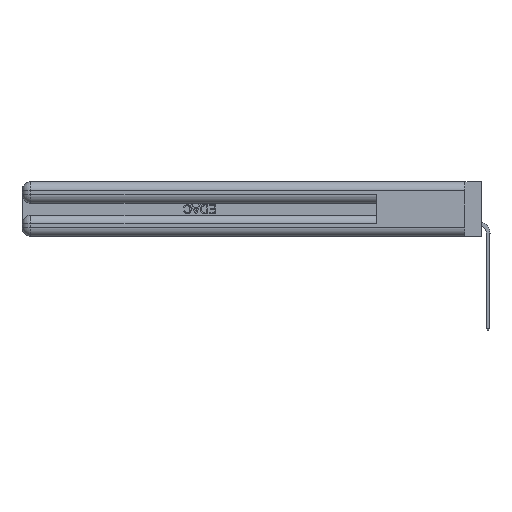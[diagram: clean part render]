
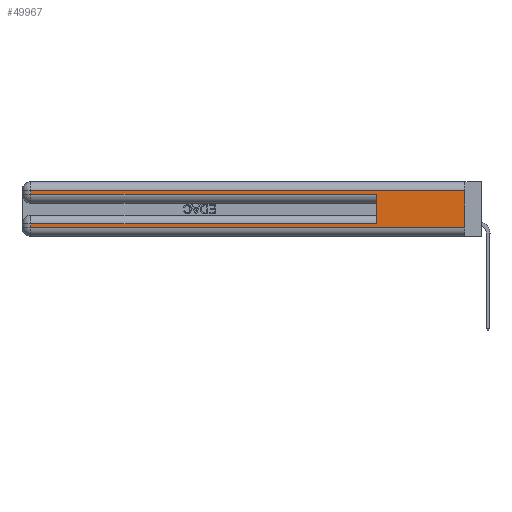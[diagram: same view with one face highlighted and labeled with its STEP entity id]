
A CAD part, left-side view. The second image highlights one B-rep face of the part: STEP entity #49967.
In plain terms, the highlighted planar face has unit normal (-1, 0, 0).
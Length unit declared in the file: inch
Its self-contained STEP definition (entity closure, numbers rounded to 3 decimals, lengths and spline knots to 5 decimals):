
#33 = CARTESIAN_POINT ( 'NONE',  ( 0., 2.94, 0.06 ) ) ;
#1053 = VERTEX_POINT ( 'NONE', #41609 ) ;
#1568 = VECTOR ( 'NONE', #34694, 39.37008 ) ;
#3211 = CARTESIAN_POINT ( 'NONE',  ( 0., 2.94, 0.37 ) ) ;
#3875 = DIRECTION ( 'NONE',  ( 0., 0., -1. ) ) ;
#4368 = EDGE_CURVE ( 'NONE', #27882, #26695, #31120, .T. ) ;
#5162 = LINE ( 'NONE', #8670, #21105 ) ;
#5306 = EDGE_CURVE ( 'NONE', #41147, #31050, #9537, .T. ) ;
#5658 = VERTEX_POINT ( 'NONE', #22631 ) ;
#6434 = ORIENTED_EDGE ( 'NONE', *, *, #20993, .F. ) ;
#6780 = ORIENTED_EDGE ( 'NONE', *, *, #15509, .T. ) ;
#6915 = DIRECTION ( 'NONE',  ( 1., 0., 0. ) ) ;
#7649 = DIRECTION ( 'NONE',  ( 0., 0., -1. ) ) ;
#8670 = CARTESIAN_POINT ( 'NONE',  ( 0., 0.6, 0.145 ) ) ;
#9537 = LINE ( 'NONE', #39548, #12088 ) ;
#10649 = EDGE_CURVE ( 'NONE', #43147, #5658, #30292, .T. ) ;
#11009 = CARTESIAN_POINT ( 'NONE',  ( 0., 0., 0.37 ) ) ;
#11147 = ORIENTED_EDGE ( 'NONE', *, *, #10649, .T. ) ;
#12088 = VECTOR ( 'NONE', #47652, 39.37008 ) ;
#12813 = EDGE_CURVE ( 'NONE', #22686, #1053, #13637, .T. ) ;
#13637 = LINE ( 'NONE', #44095, #20621 ) ;
#14068 = ORIENTED_EDGE ( 'NONE', *, *, #35236, .F. ) ;
#15509 = EDGE_CURVE ( 'NONE', #31050, #27882, #30389, .T. ) ;
#17684 = CARTESIAN_POINT ( 'NONE',  ( 0., 2.94, 0.31 ) ) ;
#18006 = ORIENTED_EDGE ( 'NONE', *, *, #21925, .T. ) ;
#18029 = LINE ( 'NONE', #46171, #1568 ) ;
#18908 = ORIENTED_EDGE ( 'NONE', *, *, #12813, .T. ) ;
#19089 = VECTOR ( 'NONE', #47805, 39.37008 ) ;
#19190 = CARTESIAN_POINT ( 'NONE',  ( 0., 2.94, 0.285 ) ) ;
#19454 = CARTESIAN_POINT ( 'NONE',  ( 0., 0., 0.285 ) ) ;
#19602 = DIRECTION ( 'NONE',  ( 0., 1., 0. ) ) ;
#20621 = VECTOR ( 'NONE', #19602, 39.37008 ) ;
#20917 = DIRECTION ( 'NONE',  ( 0., -1., 0. ) ) ;
#20993 = EDGE_CURVE ( 'NONE', #41147, #5658, #18029, .T. ) ;
#21105 = VECTOR ( 'NONE', #49849, 39.37008 ) ;
#21925 = EDGE_CURVE ( 'NONE', #1053, #43147, #50861, .T. ) ;
#22631 = CARTESIAN_POINT ( 'NONE',  ( 0., 0., 0.06 ) ) ;
#22686 = VERTEX_POINT ( 'NONE', #48046 ) ;
#23017 = DIRECTION ( 'NONE',  ( 0., 0., -1. ) ) ;
#26695 = VERTEX_POINT ( 'NONE', #37010 ) ;
#27882 = VERTEX_POINT ( 'NONE', #19190 ) ;
#30292 = LINE ( 'NONE', #47527, #32253 ) ;
#30389 = LINE ( 'NONE', #38270, #50641 ) ;
#31050 = VERTEX_POINT ( 'NONE', #17684 ) ;
#31120 = LINE ( 'NONE', #19454, #19089 ) ;
#32253 = VECTOR ( 'NONE', #20917, 39.37008 ) ;
#32547 = VECTOR ( 'NONE', #3875, 39.37008 ) ;
#34694 = DIRECTION ( 'NONE',  ( 0., 0., -1. ) ) ;
#35236 = EDGE_CURVE ( 'NONE', #22686, #26695, #5162, .T. ) ;
#35499 = ORIENTED_EDGE ( 'NONE', *, *, #4368, .T. ) ;
#37010 = CARTESIAN_POINT ( 'NONE',  ( 0., 0.6, 0.285 ) ) ;
#37459 = ORIENTED_EDGE ( 'NONE', *, *, #5306, .T. ) ;
#38270 = CARTESIAN_POINT ( 'NONE',  ( 0., 2.94, 0.37 ) ) ;
#39548 = CARTESIAN_POINT ( 'NONE',  ( 0., 0., 0.31 ) ) ;
#39807 = FACE_OUTER_BOUND ( 'NONE', #52107, .T. ) ;
#41147 = VERTEX_POINT ( 'NONE', #50049 ) ;
#41609 = CARTESIAN_POINT ( 'NONE',  ( 0., 2.94, 0.085 ) ) ;
#43147 = VERTEX_POINT ( 'NONE', #33 ) ;
#44095 = CARTESIAN_POINT ( 'NONE',  ( 0., 0., 0.085 ) ) ;
#46171 = CARTESIAN_POINT ( 'NONE',  ( 0., 0., 0.37 ) ) ;
#47527 = CARTESIAN_POINT ( 'NONE',  ( 0., 0., 0.06 ) ) ;
#47652 = DIRECTION ( 'NONE',  ( 0., 1., 0. ) ) ;
#47805 = DIRECTION ( 'NONE',  ( 0., -1., 0. ) ) ;
#48046 = CARTESIAN_POINT ( 'NONE',  ( 0., 0.6, 0.085 ) ) ;
#49849 = DIRECTION ( 'NONE',  ( 0., 0., 1. ) ) ;
#49967 = ADVANCED_FACE ( 'NONE', ( #39807 ), #51337, .F. ) ;
#50049 = CARTESIAN_POINT ( 'NONE',  ( 0., 0., 0.31 ) ) ;
#50641 = VECTOR ( 'NONE', #23017, 39.37008 ) ;
#50861 = LINE ( 'NONE', #3211, #32547 ) ;
#51337 = PLANE ( 'NONE',  #52116 ) ;
#52107 = EDGE_LOOP ( 'NONE', ( #6434, #37459, #6780, #35499, #14068, #18908, #18006, #11147 ) ) ;
#52116 = AXIS2_PLACEMENT_3D ( 'NONE', #11009, #6915, #7649 ) ;
